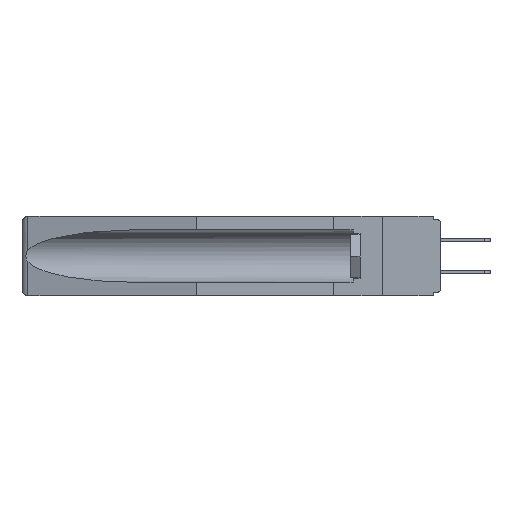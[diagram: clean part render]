
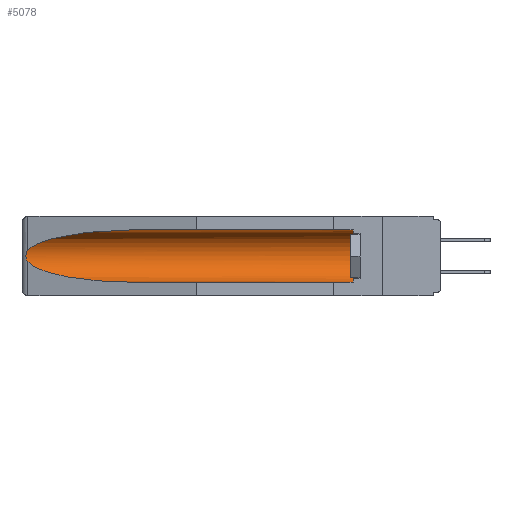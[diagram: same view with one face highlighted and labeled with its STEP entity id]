
A CAD part, left-side view. The second image highlights one B-rep face of the part: STEP entity #5078.
In plain terms, the highlighted cylindrical face has radius 2.857 mm (diameter 5.715 mm), a partial arc.
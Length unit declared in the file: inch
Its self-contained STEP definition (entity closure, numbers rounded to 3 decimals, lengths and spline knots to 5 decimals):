
#165 = CARTESIAN_POINT ( 'NONE',  ( 0.155, 0.126, -0.1715 ) ) ;
#325 =( BOUNDED_CURVE ( )  B_SPLINE_CURVE ( 3, ( #14212, #1381, #17433, #17357 ),
 .UNSPECIFIED., .F., .F. ) 
 B_SPLINE_CURVE_WITH_KNOTS ( ( 4, 4 ),
 ( 4.71239, 6.08839 ),
 .UNSPECIFIED. ) 
 CURVE ( )  GEOMETRIC_REPRESENTATION_ITEM ( )  RATIONAL_B_SPLINE_CURVE ( ( 1., 0.848, 0.848, 1. ) ) 
 REPRESENTATION_ITEM ( '' )  );
#419 = EDGE_CURVE ( 'NONE', #2819, #1705, #2790, .T. ) ;
#1381 = CARTESIAN_POINT ( 'NONE',  ( 0.21114, 1.30732, -0.059 ) ) ;
#1637 = VECTOR ( 'NONE', #4175, 39.37008 ) ;
#1705 = VERTEX_POINT ( 'NONE', #20842 ) ;
#1833 = VERTEX_POINT ( 'NONE', #11846 ) ;
#1865 = CARTESIAN_POINT ( 'NONE',  ( 0.26654, 1.53092, -0.15636 ) ) ;
#2009 = DIRECTION ( 'NONE',  ( 0., 0., 1. ) ) ;
#2127 = CARTESIAN_POINT ( 'NONE',  ( 0.155, -0.30754, -0.1715 ) ) ;
#2200 = DIRECTION ( 'NONE',  ( 0., 1., 0. ) ) ;
#2605 = ORIENTED_EDGE ( 'NONE', *, *, #419, .T. ) ;
#2790 = B_SPLINE_CURVE_WITH_KNOTS ( 'NONE', 3,
 ( #13078, #19412, #1865, #6346, #17625, #7964, #5285, #16451, #8517, #5342 ),
 .UNSPECIFIED., .F., .F.,
 ( 4, 2, 2, 2, 4 ),
 ( 0., 0.00029, 0.00058, 0.00087, 0.00117 ),
 .UNSPECIFIED. ) ;
#2819 = VERTEX_POINT ( 'NONE', #2895 ) ;
#2895 = CARTESIAN_POINT ( 'NONE',  ( 0.26537, 1.52718, -0.14972 ) ) ;
#3670 = VERTEX_POINT ( 'NONE', #17623 ) ;
#3815 = CARTESIAN_POINT ( 'NONE',  ( 0.26537, 1.52718, -0.19328 ) ) ;
#4175 = DIRECTION ( 'NONE',  ( 0., 1., 0. ) ) ;
#4554 = ORIENTED_EDGE ( 'NONE', *, *, #20304, .T. ) ;
#5078 = ADVANCED_FACE ( 'NONE', ( #16842 ), #14867, .F. ) ;
#5285 = CARTESIAN_POINT ( 'NONE',  ( 0.2673, 1.53269, -0.17917 ) ) ;
#5342 = CARTESIAN_POINT ( 'NONE',  ( 0.26537, 1.52718, -0.19328 ) ) ;
#5682 = CARTESIAN_POINT ( 'NONE',  ( 0.155, 0.126, -0.284 ) ) ;
#5981 = LINE ( 'NONE', #7528, #12019 ) ;
#6346 = CARTESIAN_POINT ( 'NONE',  ( 0.2673, 1.5327, -0.16383 ) ) ;
#6893 = CARTESIAN_POINT ( 'NONE',  ( 0.21114, 1.30732, -0.284 ) ) ;
#7260 = EDGE_CURVE ( 'NONE', #3670, #11221, #20028, .T. ) ;
#7328 = ORIENTED_EDGE ( 'NONE', *, *, #7260, .T. ) ;
#7466 = ORIENTED_EDGE ( 'NONE', *, *, #16771, .T. ) ;
#7470 = CIRCLE ( 'NONE', #14267, 0.1125 ) ;
#7528 = CARTESIAN_POINT ( 'NONE',  ( 0.155, -0.30754, -0.284 ) ) ;
#7964 = CARTESIAN_POINT ( 'NONE',  ( 0.2675, 1.53308, -0.17534 ) ) ;
#8517 = CARTESIAN_POINT ( 'NONE',  ( 0.26597, 1.5296, -0.19026 ) ) ;
#9179 = DIRECTION ( 'NONE',  ( 0., 1., 0. ) ) ;
#10754 = EDGE_LOOP ( 'NONE', ( #19166, #2605, #7466, #16712, #4554, #7328 ) ) ;
#10877 = EDGE_CURVE ( 'NONE', #13795, #1833, #5981, .T. ) ;
#11128 = CARTESIAN_POINT ( 'NONE',  ( 0.155, 1.07973, -0.059 ) ) ;
#11221 = VERTEX_POINT ( 'NONE', #11128 ) ;
#11788 = CARTESIAN_POINT ( 'NONE',  ( 0.155, -0.30754, -0.059 ) ) ;
#11846 = CARTESIAN_POINT ( 'NONE',  ( 0.155, 1.07973, -0.284 ) ) ;
#12019 = VECTOR ( 'NONE', #9179, 39.37008 ) ;
#13078 = CARTESIAN_POINT ( 'NONE',  ( 0.26537, 1.52718, -0.14972 ) ) ;
#13229 = CARTESIAN_POINT ( 'NONE',  ( 0.25451, 1.48313, -0.24835 ) ) ;
#13795 = VERTEX_POINT ( 'NONE', #5682 ) ;
#14212 = CARTESIAN_POINT ( 'NONE',  ( 0.155, 1.07973, -0.059 ) ) ;
#14267 = AXIS2_PLACEMENT_3D ( 'NONE', #165, #14425, #19351 ) ;
#14425 = DIRECTION ( 'NONE',  ( 0., -1., 0. ) ) ;
#14751 = EDGE_CURVE ( 'NONE', #11221, #2819, #325, .T. ) ;
#14867 = CYLINDRICAL_SURFACE ( 'NONE', #18759, 0.1125 ) ;
#14917 = CARTESIAN_POINT ( 'NONE',  ( 0.155, 1.07973, -0.284 ) ) ;
#16451 = CARTESIAN_POINT ( 'NONE',  ( 0.26655, 1.53094, -0.18657 ) ) ;
#16712 = ORIENTED_EDGE ( 'NONE', *, *, #10877, .F. ) ;
#16771 = EDGE_CURVE ( 'NONE', #1705, #1833, #17502, .T. ) ;
#16842 = FACE_OUTER_BOUND ( 'NONE', #10754, .T. ) ;
#17357 = CARTESIAN_POINT ( 'NONE',  ( 0.26537, 1.52718, -0.14972 ) ) ;
#17433 = CARTESIAN_POINT ( 'NONE',  ( 0.25451, 1.48313, -0.09465 ) ) ;
#17502 =( BOUNDED_CURVE ( )  B_SPLINE_CURVE ( 3, ( #3815, #13229, #6893, #14917 ),
 .UNSPECIFIED., .F., .F. ) 
 B_SPLINE_CURVE_WITH_KNOTS ( ( 4, 4 ),
 ( 0.1948, 1.5708 ),
 .UNSPECIFIED. ) 
 CURVE ( )  GEOMETRIC_REPRESENTATION_ITEM ( )  RATIONAL_B_SPLINE_CURVE ( ( 1., 0.848, 0.848, 1. ) ) 
 REPRESENTATION_ITEM ( '' )  );
#17623 = CARTESIAN_POINT ( 'NONE',  ( 0.155, 0.126, -0.059 ) ) ;
#17625 = CARTESIAN_POINT ( 'NONE',  ( 0.2675, 1.53308, -0.16763 ) ) ;
#18759 = AXIS2_PLACEMENT_3D ( 'NONE', #2127, #2200, #2009 ) ;
#19166 = ORIENTED_EDGE ( 'NONE', *, *, #14751, .T. ) ;
#19351 = DIRECTION ( 'NONE',  ( 0., 0., 1. ) ) ;
#19412 = CARTESIAN_POINT ( 'NONE',  ( 0.26597, 1.52961, -0.15275 ) ) ;
#20028 = LINE ( 'NONE', #11788, #1637 ) ;
#20304 = EDGE_CURVE ( 'NONE', #13795, #3670, #7470, .T. ) ;
#20842 = CARTESIAN_POINT ( 'NONE',  ( 0.26537, 1.52718, -0.19328 ) ) ;
